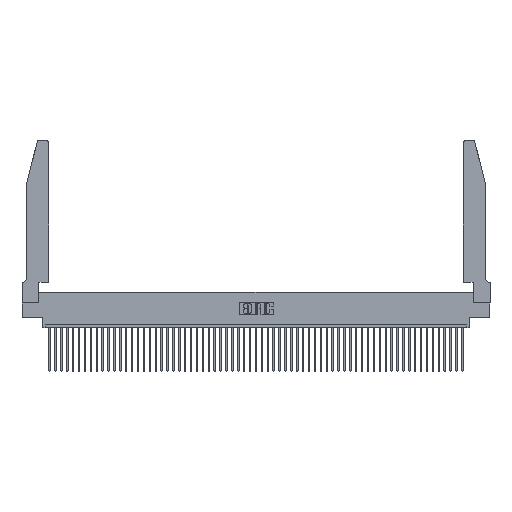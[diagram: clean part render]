
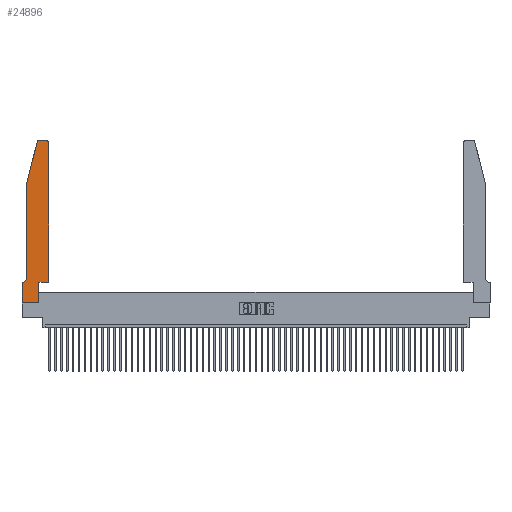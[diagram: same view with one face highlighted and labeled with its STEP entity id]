
A CAD part, top view. The second image highlights one B-rep face of the part: STEP entity #24896.
In plain terms, the highlighted planar face has unit normal (0, 0, 1).
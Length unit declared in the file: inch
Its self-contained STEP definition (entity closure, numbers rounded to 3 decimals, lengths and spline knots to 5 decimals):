
#1339 = CARTESIAN_POINT ( 'NONE',  ( 0.284, 2.72, 0.37 ) ) ;
#2025 = CARTESIAN_POINT ( 'NONE',  ( 0.4205, 2.72, 0.37 ) ) ;
#4530 = EDGE_CURVE ( 'NONE', #47301, #9775, #9233, .T. ) ;
#4880 = AXIS2_PLACEMENT_3D ( 'NONE', #1339, #43124, #39078 ) ;
#5173 = LINE ( 'NONE', #7310, #28608 ) ;
#5779 = VECTOR ( 'NONE', #35274, 39.37008 ) ;
#5870 = CARTESIAN_POINT ( 'NONE',  ( 0., 0., 0.37 ) ) ;
#6495 = ORIENTED_EDGE ( 'NONE', *, *, #34267, .T. ) ;
#7204 = DIRECTION ( 'NONE',  ( 0., 1., 0. ) ) ;
#7310 = CARTESIAN_POINT ( 'NONE',  ( 0., 0., 0.37 ) ) ;
#8500 = CARTESIAN_POINT ( 'NONE',  ( 0.0055, 0.35, 0.37 ) ) ;
#8671 = DIRECTION ( 'NONE',  ( -1., 0., 0. ) ) ;
#9134 = FACE_OUTER_BOUND ( 'NONE', #52950, .T. ) ;
#9233 = LINE ( 'NONE', #12913, #9882 ) ;
#9265 = EDGE_CURVE ( 'NONE', #41880, #28575, #53379, .T. ) ;
#9775 = VERTEX_POINT ( 'NONE', #36637 ) ;
#9882 = VECTOR ( 'NONE', #51789, 39.37008 ) ;
#10033 = DIRECTION ( 'NONE',  ( 0., -1., 0. ) ) ;
#11659 = DIRECTION ( 'NONE',  ( 1., 0., 0. ) ) ;
#12036 = CARTESIAN_POINT ( 'NONE',  ( 0.4205, 2.75, 0.37 ) ) ;
#12913 = CARTESIAN_POINT ( 'NONE',  ( 0.0755, 2., 0.37 ) ) ;
#13913 = VERTEX_POINT ( 'NONE', #19219 ) ;
#14203 = CARTESIAN_POINT ( 'NONE',  ( 0.2865, 0.35, 0.37 ) ) ;
#15113 = CARTESIAN_POINT ( 'NONE',  ( 0.0055, 0.42, 0.37 ) ) ;
#15209 = VECTOR ( 'NONE', #7204, 39.37008 ) ;
#15277 = VECTOR ( 'NONE', #8671, 39.37008 ) ;
#15370 = VERTEX_POINT ( 'NONE', #31460 ) ;
#15614 = VECTOR ( 'NONE', #21188, 39.37008 ) ;
#16591 = CARTESIAN_POINT ( 'NONE',  ( 0.2605, 2.75, 0.37 ) ) ;
#16754 = VERTEX_POINT ( 'NONE', #18434 ) ;
#17069 = CARTESIAN_POINT ( 'NONE',  ( 0.0755, 0.35, 0.37 ) ) ;
#17626 = EDGE_CURVE ( 'NONE', #45073, #16754, #48795, .T. ) ;
#18017 = PLANE ( 'NONE',  #46522 ) ;
#18229 = LINE ( 'NONE', #20756, #5779 ) ;
#18434 = CARTESIAN_POINT ( 'NONE',  ( 0.2865, 0.35, 0.37 ) ) ;
#18975 = VERTEX_POINT ( 'NONE', #33770 ) ;
#19219 = CARTESIAN_POINT ( 'NONE',  ( 0.25487, 2.72718, 0.37 ) ) ;
#19381 = DIRECTION ( 'NONE',  ( -1., 0., 0. ) ) ;
#19605 = ORIENTED_EDGE ( 'NONE', *, *, #50111, .T. ) ;
#19978 = EDGE_CURVE ( 'NONE', #15370, #41880, #18229, .T. ) ;
#20361 = CARTESIAN_POINT ( 'NONE',  ( 0.0755, 2., 0.37 ) ) ;
#20368 = DIRECTION ( 'NONE',  ( -1., 0., 0. ) ) ;
#20491 = EDGE_CURVE ( 'NONE', #32292, #45073, #5173, .T. ) ;
#20643 = ORIENTED_EDGE ( 'NONE', *, *, #19978, .T. ) ;
#20756 = CARTESIAN_POINT ( 'NONE',  ( 0.4505, 0.35, 0.37 ) ) ;
#21040 = VERTEX_POINT ( 'NONE', #23993 ) ;
#21109 = CARTESIAN_POINT ( 'NONE',  ( 0., 0., 0.37 ) ) ;
#21188 = DIRECTION ( 'NONE',  ( -0.239, -0.971, 0. ) ) ;
#21315 = VECTOR ( 'NONE', #24256, 39.37008 ) ;
#22320 = ORIENTED_EDGE ( 'NONE', *, *, #20491, .T. ) ;
#22456 = DIRECTION ( 'NONE',  ( 0., 0., 1. ) ) ;
#23993 = CARTESIAN_POINT ( 'NONE',  ( 0., 0.35, 0.37 ) ) ;
#24256 = DIRECTION ( 'NONE',  ( 1., 0., 0. ) ) ;
#24896 = ADVANCED_FACE ( 'NONE', ( #9134 ), #18017, .T. ) ;
#25270 = CARTESIAN_POINT ( 'NONE',  ( 0.0755, 2., 0.37 ) ) ;
#26411 = LINE ( 'NONE', #17069, #15277 ) ;
#28307 = CARTESIAN_POINT ( 'NONE',  ( 0.4505, 0.35, 0.37 ) ) ;
#28575 = VERTEX_POINT ( 'NONE', #12036 ) ;
#28608 = VECTOR ( 'NONE', #11659, 39.37008 ) ;
#31303 = LINE ( 'NONE', #25270, #15614 ) ;
#31460 = CARTESIAN_POINT ( 'NONE',  ( 0.4505, 0.35, 0.37 ) ) ;
#32292 = VERTEX_POINT ( 'NONE', #21109 ) ;
#33770 = CARTESIAN_POINT ( 'NONE',  ( 0.284, 2.75, 0.37 ) ) ;
#33935 = AXIS2_PLACEMENT_3D ( 'NONE', #2025, #47391, #47581 ) ;
#34005 = EDGE_CURVE ( 'NONE', #21040, #32292, #44604, .T. ) ;
#34267 = EDGE_CURVE ( 'NONE', #9775, #39927, #37445, .T. ) ;
#34509 = ORIENTED_EDGE ( 'NONE', *, *, #4530, .T. ) ;
#34686 = EDGE_CURVE ( 'NONE', #18975, #13913, #38038, .T. ) ;
#35143 = ORIENTED_EDGE ( 'NONE', *, *, #34686, .T. ) ;
#35159 = DIRECTION ( 'NONE',  ( 1., 0., 0. ) ) ;
#35274 = DIRECTION ( 'NONE',  ( 0., 1., 0. ) ) ;
#35373 = EDGE_CURVE ( 'NONE', #13913, #47301, #31303, .T. ) ;
#36149 = ORIENTED_EDGE ( 'NONE', *, *, #9265, .T. ) ;
#36470 = ORIENTED_EDGE ( 'NONE', *, *, #41043, .T. ) ;
#36637 = CARTESIAN_POINT ( 'NONE',  ( 0.0755, 0.42, 0.37 ) ) ;
#37373 = ORIENTED_EDGE ( 'NONE', *, *, #41811, .T. ) ;
#37445 = CIRCLE ( 'NONE', #40871, 0.07 ) ;
#38038 = CIRCLE ( 'NONE', #4880, 0.03 ) ;
#39078 = DIRECTION ( 'NONE',  ( 1., 0., 0. ) ) ;
#39192 = CARTESIAN_POINT ( 'NONE',  ( 0.2865, 0., 0.37 ) ) ;
#39927 = VERTEX_POINT ( 'NONE', #8500 ) ;
#40574 = ORIENTED_EDGE ( 'NONE', *, *, #17626, .T. ) ;
#40871 = AXIS2_PLACEMENT_3D ( 'NONE', #15113, #44566, #19381 ) ;
#41043 = EDGE_CURVE ( 'NONE', #16754, #15370, #46334, .T. ) ;
#41811 = EDGE_CURVE ( 'NONE', #39927, #21040, #26411, .T. ) ;
#41880 = VERTEX_POINT ( 'NONE', #54316 ) ;
#43124 = DIRECTION ( 'NONE',  ( 0., 0., 1. ) ) ;
#43557 = ORIENTED_EDGE ( 'NONE', *, *, #35373, .T. ) ;
#44448 = ORIENTED_EDGE ( 'NONE', *, *, #34005, .T. ) ;
#44566 = DIRECTION ( 'NONE',  ( 0., 0., -1. ) ) ;
#44604 = LINE ( 'NONE', #5870, #51723 ) ;
#45073 = VERTEX_POINT ( 'NONE', #39192 ) ;
#46334 = LINE ( 'NONE', #28307, #21315 ) ;
#46522 = AXIS2_PLACEMENT_3D ( 'NONE', #51865, #22456, #35159 ) ;
#47301 = VERTEX_POINT ( 'NONE', #20361 ) ;
#47391 = DIRECTION ( 'NONE',  ( 0., 0., 1. ) ) ;
#47581 = DIRECTION ( 'NONE',  ( 1., 0., 0. ) ) ;
#48696 = LINE ( 'NONE', #16591, #51263 ) ;
#48795 = LINE ( 'NONE', #14203, #15209 ) ;
#50111 = EDGE_CURVE ( 'NONE', #28575, #18975, #48696, .T. ) ;
#51263 = VECTOR ( 'NONE', #20368, 39.37008 ) ;
#51723 = VECTOR ( 'NONE', #10033, 39.37008 ) ;
#51789 = DIRECTION ( 'NONE',  ( 0., -1., 0. ) ) ;
#51865 = CARTESIAN_POINT ( 'NONE',  ( 0., 0.35, 0.37 ) ) ;
#52950 = EDGE_LOOP ( 'NONE', ( #19605, #35143, #43557, #34509, #6495, #37373, #44448, #22320, #40574, #36470, #20643, #36149 ) ) ;
#53379 = CIRCLE ( 'NONE', #33935, 0.03 ) ;
#54316 = CARTESIAN_POINT ( 'NONE',  ( 0.4505, 2.72, 0.37 ) ) ;
